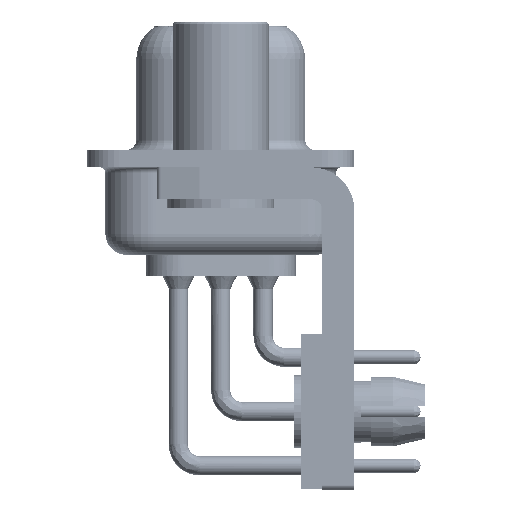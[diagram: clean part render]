
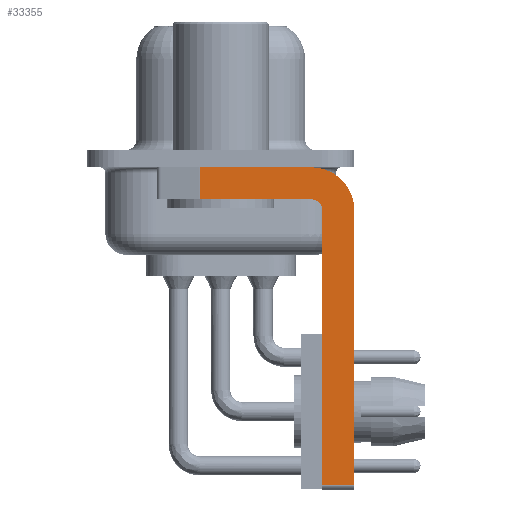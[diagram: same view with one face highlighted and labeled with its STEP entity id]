
A CAD part, left-side view. The second image highlights one B-rep face of the part: STEP entity #33355.
In plain terms, the highlighted planar face has unit normal (-1, 0, 0).
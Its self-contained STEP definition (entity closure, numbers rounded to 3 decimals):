
#606 = FACE_OUTER_BOUND ( 'NONE', #40239, .T. ) ;
#646 = ORIENTED_EDGE ( 'NONE', *, *, #41755, .F. ) ;
#1383 = CARTESIAN_POINT ( 'NONE',  ( -2.9, 3., -0.4 ) ) ;
#2508 = EDGE_CURVE ( 'NONE', #38887, #38720, #37917, .T. ) ;
#2935 = VERTEX_POINT ( 'NONE', #11486 ) ;
#5463 = ORIENTED_EDGE ( 'NONE', *, *, #7138, .T. ) ;
#7138 = EDGE_CURVE ( 'NONE', #41590, #38720, #38205, .T. ) ;
#7488 = CIRCLE ( 'NONE', #27178, 0.5 ) ;
#10277 = PLANE ( 'NONE',  #32881 ) ;
#10897 = DIRECTION ( 'NONE',  ( 1., 0., 0. ) ) ;
#10909 = VECTOR ( 'NONE', #42211, 1000. ) ;
#11005 = ORIENTED_EDGE ( 'NONE', *, *, #24179, .F. ) ;
#11086 = CIRCLE ( 'NONE', #46392, 2. ) ;
#11486 = CARTESIAN_POINT ( 'NONE',  ( -2.9, -6.25, -2.4 ) ) ;
#13911 = DIRECTION ( 'NONE',  ( 0., 0., -1. ) ) ;
#14797 = CARTESIAN_POINT ( 'NONE',  ( -2.9, -4.25, -0.4 ) ) ;
#14891 = CARTESIAN_POINT ( 'NONE',  ( -2.9, 0.978, -0.4 ) ) ;
#15596 = VERTEX_POINT ( 'NONE', #26039 ) ;
#17248 = CARTESIAN_POINT ( 'NONE',  ( -2.9, -4.25, -15.25 ) ) ;
#17383 = ORIENTED_EDGE ( 'NONE', *, *, #19140, .F. ) ;
#18027 = CARTESIAN_POINT ( 'NONE',  ( -2.9, -4.75, -15.5 ) ) ;
#19140 = EDGE_CURVE ( 'NONE', #41590, #34951, #22795, .T. ) ;
#19545 = CARTESIAN_POINT ( 'NONE',  ( -2.9, -4.25, -2.4 ) ) ;
#19860 = LINE ( 'NONE', #17248, #22059 ) ;
#21534 = EDGE_CURVE ( 'NONE', #36430, #39456, #19860, .T. ) ;
#21680 = EDGE_CURVE ( 'NONE', #36430, #15596, #26977, .T. ) ;
#22059 = VECTOR ( 'NONE', #38653, 1000. ) ;
#22795 = LINE ( 'NONE', #1383, #30036 ) ;
#22902 = DIRECTION ( 'NONE',  ( 0., -1., 0. ) ) ;
#23030 = DIRECTION ( 'NONE',  ( 0., 0., 1. ) ) ;
#24179 = EDGE_CURVE ( 'NONE', #2935, #39456, #41749, .T. ) ;
#26039 = CARTESIAN_POINT ( 'NONE',  ( -2.9, -4.75, -2.4 ) ) ;
#26977 = LINE ( 'NONE', #18027, #42731 ) ;
#27178 = AXIS2_PLACEMENT_3D ( 'NONE', #19545, #44517, #23030 ) ;
#27601 = CARTESIAN_POINT ( 'NONE',  ( -2.9, -6.25, -2.4 ) ) ;
#27778 = ORIENTED_EDGE ( 'NONE', *, *, #2508, .F. ) ;
#28379 = VECTOR ( 'NONE', #37911, 1000. ) ;
#30036 = VECTOR ( 'NONE', #22902, 1000. ) ;
#31228 = DIRECTION ( 'NONE',  ( 0., 0., -1. ) ) ;
#32219 = CARTESIAN_POINT ( 'NONE',  ( -2.9, -4.25, -2.4 ) ) ;
#32779 = CARTESIAN_POINT ( 'NONE',  ( -2.9, 0.978, -1.9 ) ) ;
#32881 = AXIS2_PLACEMENT_3D ( 'NONE', #45952, #35207, #13911 ) ;
#33171 = CARTESIAN_POINT ( 'NONE',  ( -2.9, -6.25, -15.25 ) ) ;
#33355 = ADVANCED_FACE ( 'NONE', ( #606 ), #10277, .F. ) ;
#34951 = VERTEX_POINT ( 'NONE', #14797 ) ;
#35207 = DIRECTION ( 'NONE',  ( 1., 0., 0. ) ) ;
#35801 = DIRECTION ( 'NONE',  ( 0., 0., -1. ) ) ;
#36430 = VERTEX_POINT ( 'NONE', #40022 ) ;
#36831 = ORIENTED_EDGE ( 'NONE', *, *, #21680, .F. ) ;
#37071 = ORIENTED_EDGE ( 'NONE', *, *, #44012, .F. ) ;
#37153 = CARTESIAN_POINT ( 'NONE',  ( -2.9, -4.25, -1.9 ) ) ;
#37911 = DIRECTION ( 'NONE',  ( 0., 1., 0. ) ) ;
#37917 = LINE ( 'NONE', #39824, #28379 ) ;
#38205 = LINE ( 'NONE', #38588, #10909 ) ;
#38588 = CARTESIAN_POINT ( 'NONE',  ( -2.9, 0.978, -1.9 ) ) ;
#38653 = DIRECTION ( 'NONE',  ( 0., -1., 0. ) ) ;
#38720 = VERTEX_POINT ( 'NONE', #32779 ) ;
#38887 = VERTEX_POINT ( 'NONE', #37153 ) ;
#39456 = VERTEX_POINT ( 'NONE', #33171 ) ;
#39824 = CARTESIAN_POINT ( 'NONE',  ( -2.9, -4.25, -1.9 ) ) ;
#40022 = CARTESIAN_POINT ( 'NONE',  ( -2.9, -4.75, -15.25 ) ) ;
#40239 = EDGE_LOOP ( 'NONE', ( #17383, #5463, #27778, #646, #36831, #42006, #11005, #37071 ) ) ;
#40625 = VECTOR ( 'NONE', #31228, 1000. ) ;
#41590 = VERTEX_POINT ( 'NONE', #14891 ) ;
#41749 = LINE ( 'NONE', #27601, #40625 ) ;
#41755 = EDGE_CURVE ( 'NONE', #15596, #38887, #7488, .T. ) ;
#42006 = ORIENTED_EDGE ( 'NONE', *, *, #21534, .T. ) ;
#42211 = DIRECTION ( 'NONE',  ( 0., 0., -1. ) ) ;
#42731 = VECTOR ( 'NONE', #42942, 1000. ) ;
#42942 = DIRECTION ( 'NONE',  ( 0., 0., 1. ) ) ;
#44012 = EDGE_CURVE ( 'NONE', #34951, #2935, #11086, .T. ) ;
#44517 = DIRECTION ( 'NONE',  ( -1., 0., 0. ) ) ;
#45952 = CARTESIAN_POINT ( 'NONE',  ( -2.9, -4.25, -2.4 ) ) ;
#46392 = AXIS2_PLACEMENT_3D ( 'NONE', #32219, #10897, #35801 ) ;
